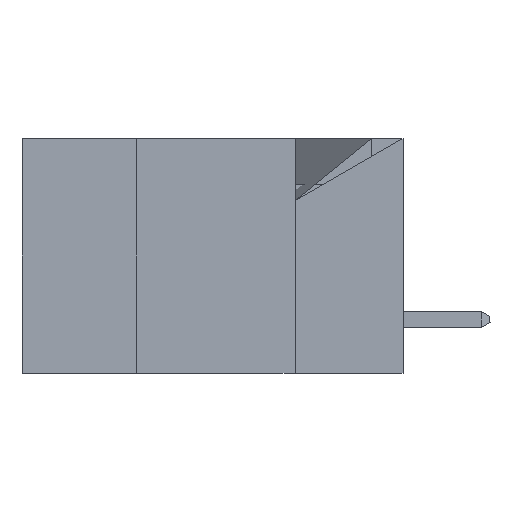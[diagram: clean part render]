
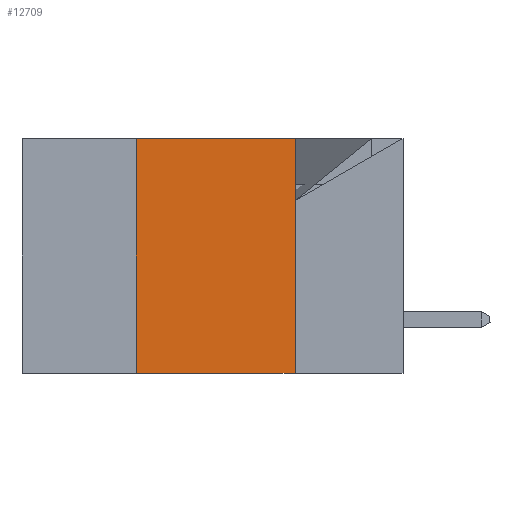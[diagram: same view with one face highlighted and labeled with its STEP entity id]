
A CAD part, left-side view. The second image highlights one B-rep face of the part: STEP entity #12709.
In plain terms, the highlighted planar face has unit normal (-1, 0, 0).
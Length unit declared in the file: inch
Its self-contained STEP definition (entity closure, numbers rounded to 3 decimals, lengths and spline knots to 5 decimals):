
#1061 = DIRECTION ( 'NONE',  ( 0., 0., 1. ) ) ;
#1152 = ORIENTED_EDGE ( 'NONE', *, *, #16746, .F. ) ;
#1691 = FACE_OUTER_BOUND ( 'NONE', #8384, .T. ) ;
#1949 = VECTOR ( 'NONE', #4352, 39.37008 ) ;
#2332 = DIRECTION ( 'NONE',  ( 0., -1., 0. ) ) ;
#2515 = CARTESIAN_POINT ( 'NONE',  ( 0., 0.42, -0.37 ) ) ;
#2937 = CARTESIAN_POINT ( 'NONE',  ( 0., 0.17, 0. ) ) ;
#3344 = EDGE_CURVE ( 'NONE', #10885, #16554, #12741, .T. ) ;
#3812 = CARTESIAN_POINT ( 'NONE',  ( 0., 0.6, -0.37 ) ) ;
#4352 = DIRECTION ( 'NONE',  ( 0., 0., -1. ) ) ;
#4716 = ORIENTED_EDGE ( 'NONE', *, *, #11054, .F. ) ;
#5253 = LINE ( 'NONE', #14257, #15057 ) ;
#5349 = DIRECTION ( 'NONE',  ( 1., 0., 0. ) ) ;
#5467 = VECTOR ( 'NONE', #6039, 39.37008 ) ;
#6039 = DIRECTION ( 'NONE',  ( 0., -1., 0. ) ) ;
#7549 = CARTESIAN_POINT ( 'NONE',  ( 0., 0.17, -0.37 ) ) ;
#7730 = LINE ( 'NONE', #16494, #14094 ) ;
#7814 = CARTESIAN_POINT ( 'NONE',  ( 0., 0.17, 0. ) ) ;
#7952 = ORIENTED_EDGE ( 'NONE', *, *, #3344, .T. ) ;
#8351 = ORIENTED_EDGE ( 'NONE', *, *, #10091, .F. ) ;
#8384 = EDGE_LOOP ( 'NONE', ( #4716, #8351, #1152, #7952 ) ) ;
#9066 = LINE ( 'NONE', #2937, #1949 ) ;
#10091 = EDGE_CURVE ( 'NONE', #10843, #10845, #7730, .T. ) ;
#10843 = VERTEX_POINT ( 'NONE', #16607 ) ;
#10845 = VERTEX_POINT ( 'NONE', #7814 ) ;
#10885 = VERTEX_POINT ( 'NONE', #2515 ) ;
#11054 = EDGE_CURVE ( 'NONE', #10845, #16554, #9066, .T. ) ;
#12709 = ADVANCED_FACE ( 'NONE', ( #1691 ), #13063, .F. ) ;
#12741 = LINE ( 'NONE', #3812, #5467 ) ;
#12956 = CARTESIAN_POINT ( 'NONE',  ( 0., 0.6, 0. ) ) ;
#13063 = PLANE ( 'NONE',  #14100 ) ;
#14094 = VECTOR ( 'NONE', #2332, 39.37008 ) ;
#14100 = AXIS2_PLACEMENT_3D ( 'NONE', #12956, #5349, #14327 ) ;
#14257 = CARTESIAN_POINT ( 'NONE',  ( 0., 0.42, 0. ) ) ;
#14327 = DIRECTION ( 'NONE',  ( 0., 0., -1. ) ) ;
#15057 = VECTOR ( 'NONE', #1061, 39.37008 ) ;
#16494 = CARTESIAN_POINT ( 'NONE',  ( 0., 0.6, 0. ) ) ;
#16554 = VERTEX_POINT ( 'NONE', #7549 ) ;
#16607 = CARTESIAN_POINT ( 'NONE',  ( 0., 0.42, 0. ) ) ;
#16746 = EDGE_CURVE ( 'NONE', #10885, #10843, #5253, .T. ) ;
